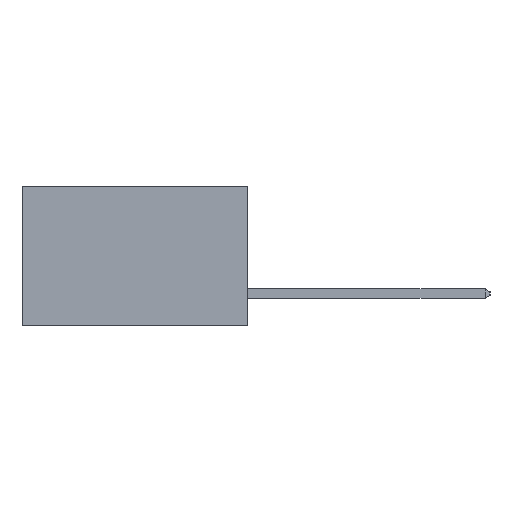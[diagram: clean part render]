
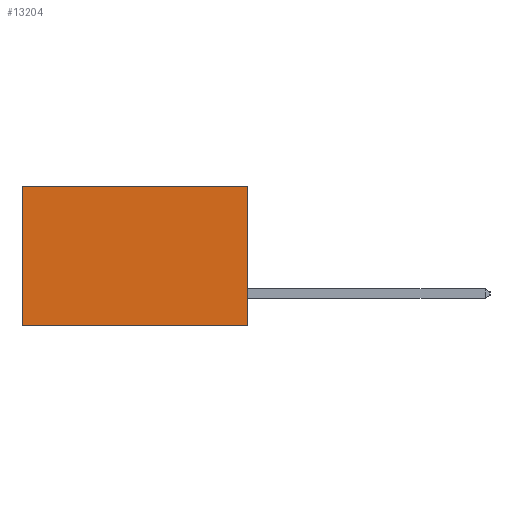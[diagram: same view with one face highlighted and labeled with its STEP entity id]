
A CAD part, left-side view. The second image highlights one B-rep face of the part: STEP entity #13204.
In plain terms, the highlighted planar face has unit normal (-1, 0, 0).
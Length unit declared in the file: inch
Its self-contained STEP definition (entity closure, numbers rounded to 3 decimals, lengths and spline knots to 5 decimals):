
#105 = DIRECTION ( 'NONE',  ( 0., 0., -1. ) ) ;
#131 = DIRECTION ( 'NONE',  ( 1., 0., 0. ) ) ;
#275 = CARTESIAN_POINT ( 'NONE',  ( 0.2615, 0., -0.37 ) ) ;
#434 = PLANE ( 'NONE',  #10625 ) ;
#696 = LINE ( 'NONE', #17924, #4358 ) ;
#1194 = VECTOR ( 'NONE', #13167, 39.37008 ) ;
#1826 = CARTESIAN_POINT ( 'NONE',  ( 0.2615, 0., 0. ) ) ;
#2618 = VECTOR ( 'NONE', #9370, 39.37008 ) ;
#2983 = CARTESIAN_POINT ( 'NONE',  ( 0.2615, 0.6, 0. ) ) ;
#4178 = VECTOR ( 'NONE', #16588, 39.37008 ) ;
#4358 = VECTOR ( 'NONE', #10586, 39.37008 ) ;
#5008 = EDGE_CURVE ( 'NONE', #5389, #18744, #15919, .T. ) ;
#5389 = VERTEX_POINT ( 'NONE', #1826 ) ;
#7362 = LINE ( 'NONE', #16838, #2618 ) ;
#7467 = EDGE_LOOP ( 'NONE', ( #10419, #14954, #9203, #8639 ) ) ;
#8639 = ORIENTED_EDGE ( 'NONE', *, *, #5008, .T. ) ;
#9203 = ORIENTED_EDGE ( 'NONE', *, *, #16164, .F. ) ;
#9370 = DIRECTION ( 'NONE',  ( 0., 1., 0. ) ) ;
#9558 = LINE ( 'NONE', #12858, #1194 ) ;
#9774 = VERTEX_POINT ( 'NONE', #16174 ) ;
#9936 = EDGE_CURVE ( 'NONE', #18744, #11379, #9558, .T. ) ;
#10419 = ORIENTED_EDGE ( 'NONE', *, *, #9936, .T. ) ;
#10586 = DIRECTION ( 'NONE',  ( 0., 0., -1. ) ) ;
#10625 = AXIS2_PLACEMENT_3D ( 'NONE', #275, #131, #105 ) ;
#11181 = CARTESIAN_POINT ( 'NONE',  ( 0.2615, 0.6, -0.37 ) ) ;
#11379 = VERTEX_POINT ( 'NONE', #11181 ) ;
#12858 = CARTESIAN_POINT ( 'NONE',  ( 0.2615, 0.6, -0.37 ) ) ;
#13167 = DIRECTION ( 'NONE',  ( 0., 0., -1. ) ) ;
#13204 = ADVANCED_FACE ( 'NONE', ( #15978 ), #434, .F. ) ;
#14954 = ORIENTED_EDGE ( 'NONE', *, *, #15637, .F. ) ;
#15637 = EDGE_CURVE ( 'NONE', #9774, #11379, #7362, .T. ) ;
#15919 = LINE ( 'NONE', #16552, #4178 ) ;
#15978 = FACE_OUTER_BOUND ( 'NONE', #7467, .T. ) ;
#16164 = EDGE_CURVE ( 'NONE', #5389, #9774, #696, .T. ) ;
#16174 = CARTESIAN_POINT ( 'NONE',  ( 0.2615, 0., -0.37 ) ) ;
#16552 = CARTESIAN_POINT ( 'NONE',  ( 0.2615, 0., 0. ) ) ;
#16588 = DIRECTION ( 'NONE',  ( 0., 1., 0. ) ) ;
#16838 = CARTESIAN_POINT ( 'NONE',  ( 0.2615, 0., -0.37 ) ) ;
#17924 = CARTESIAN_POINT ( 'NONE',  ( 0.2615, 0., -0.37 ) ) ;
#18744 = VERTEX_POINT ( 'NONE', #2983 ) ;
